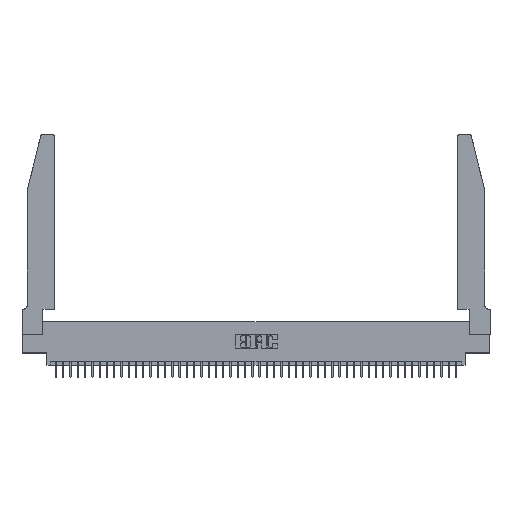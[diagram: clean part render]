
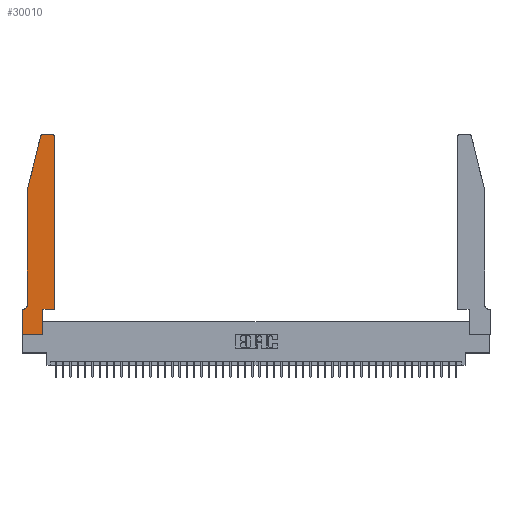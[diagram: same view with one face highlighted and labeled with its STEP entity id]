
A CAD part, top view. The second image highlights one B-rep face of the part: STEP entity #30010.
In plain terms, the highlighted planar face has unit normal (0, 0, 1).
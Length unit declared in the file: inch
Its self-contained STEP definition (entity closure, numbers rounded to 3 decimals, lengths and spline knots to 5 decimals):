
#52 = CARTESIAN_POINT ( 'NONE',  ( 0.4205, 2.75, 0.37 ) ) ;
#206 = VECTOR ( 'NONE', #19448, 39.37008 ) ;
#231 = VECTOR ( 'NONE', #16104, 39.37008 ) ;
#525 = LINE ( 'NONE', #16899, #36993 ) ;
#2098 = EDGE_CURVE ( 'NONE', #26644, #42607, #46910, .T. ) ;
#2677 = DIRECTION ( 'NONE',  ( 0., 0., -1. ) ) ;
#2873 = CARTESIAN_POINT ( 'NONE',  ( 0., 0., 0.37 ) ) ;
#5115 = VERTEX_POINT ( 'NONE', #46144 ) ;
#5498 = CARTESIAN_POINT ( 'NONE',  ( 0.284, 2.75, 0.37 ) ) ;
#6002 = AXIS2_PLACEMENT_3D ( 'NONE', #24562, #2677, #28212 ) ;
#6531 = ORIENTED_EDGE ( 'NONE', *, *, #21358, .T. ) ;
#7014 = CARTESIAN_POINT ( 'NONE',  ( 0., 0.35, 0.37 ) ) ;
#8141 = DIRECTION ( 'NONE',  ( 0., 1., 0. ) ) ;
#8501 = DIRECTION ( 'NONE',  ( 1., 0., 0. ) ) ;
#8911 = LINE ( 'NONE', #37451, #206 ) ;
#9303 = ORIENTED_EDGE ( 'NONE', *, *, #23251, .T. ) ;
#9736 = DIRECTION ( 'NONE',  ( 1., 0., 0. ) ) ;
#9850 = CARTESIAN_POINT ( 'NONE',  ( 0.0055, 0.35, 0.37 ) ) ;
#10050 = CARTESIAN_POINT ( 'NONE',  ( 0.4505, 2.72, 0.37 ) ) ;
#10442 = DIRECTION ( 'NONE',  ( -0.239, -0.971, 0. ) ) ;
#10679 = DIRECTION ( 'NONE',  ( 1., 0., 0. ) ) ;
#12460 = CARTESIAN_POINT ( 'NONE',  ( 0.2605, 2.75, 0.37 ) ) ;
#12537 = LINE ( 'NONE', #18976, #39134 ) ;
#13450 = CARTESIAN_POINT ( 'NONE',  ( 0.2865, 0., 0.37 ) ) ;
#15538 = VERTEX_POINT ( 'NONE', #2873 ) ;
#16104 = DIRECTION ( 'NONE',  ( -1., 0., 0. ) ) ;
#16208 = VERTEX_POINT ( 'NONE', #10050 ) ;
#16347 = CARTESIAN_POINT ( 'NONE',  ( 0.284, 2.72, 0.37 ) ) ;
#16579 = LINE ( 'NONE', #35060, #44237 ) ;
#16899 = CARTESIAN_POINT ( 'NONE',  ( 0., 0., 0.37 ) ) ;
#17254 = DIRECTION ( 'NONE',  ( 0., 0., 1. ) ) ;
#17348 = ORIENTED_EDGE ( 'NONE', *, *, #21017, .T. ) ;
#17384 = EDGE_CURVE ( 'NONE', #24950, #5115, #42437, .T. ) ;
#18054 = CARTESIAN_POINT ( 'NONE',  ( 0.2865, 0.35, 0.37 ) ) ;
#18840 = ORIENTED_EDGE ( 'NONE', *, *, #28044, .T. ) ;
#18976 = CARTESIAN_POINT ( 'NONE',  ( 0.2865, 0.35, 0.37 ) ) ;
#19448 = DIRECTION ( 'NONE',  ( -1., 0., 0. ) ) ;
#19461 = CIRCLE ( 'NONE', #28819, 0.03 ) ;
#19808 = ORIENTED_EDGE ( 'NONE', *, *, #28953, .T. ) ;
#20025 = DIRECTION ( 'NONE',  ( 1., 0., 0. ) ) ;
#20196 = VERTEX_POINT ( 'NONE', #38527 ) ;
#20366 = CARTESIAN_POINT ( 'NONE',  ( 0., 0.35, 0.37 ) ) ;
#20923 = LINE ( 'NONE', #12460, #231 ) ;
#21017 = EDGE_CURVE ( 'NONE', #16208, #32148, #25119, .T. ) ;
#21186 = EDGE_LOOP ( 'NONE', ( #9303, #39780, #45059, #41513, #21850, #19808, #25173, #21881, #6531, #23293, #18840, #17348 ) ) ;
#21194 = LINE ( 'NONE', #42920, #38115 ) ;
#21358 = EDGE_CURVE ( 'NONE', #45138, #24950, #12537, .T. ) ;
#21850 = ORIENTED_EDGE ( 'NONE', *, *, #23458, .T. ) ;
#21881 = ORIENTED_EDGE ( 'NONE', *, *, #25416, .T. ) ;
#23251 = EDGE_CURVE ( 'NONE', #32148, #41330, #20923, .T. ) ;
#23293 = ORIENTED_EDGE ( 'NONE', *, *, #17384, .T. ) ;
#23458 = EDGE_CURVE ( 'NONE', #20196, #37422, #41261, .T. ) ;
#24562 = CARTESIAN_POINT ( 'NONE',  ( 0.0055, 0.42, 0.37 ) ) ;
#24950 = VERTEX_POINT ( 'NONE', #18054 ) ;
#25119 = CIRCLE ( 'NONE', #32746, 0.03 ) ;
#25173 = ORIENTED_EDGE ( 'NONE', *, *, #37398, .T. ) ;
#25416 = EDGE_CURVE ( 'NONE', #15538, #45138, #525, .T. ) ;
#25746 = CARTESIAN_POINT ( 'NONE',  ( 0.4505, 0.35, 0.37 ) ) ;
#26644 = VERTEX_POINT ( 'NONE', #45790 ) ;
#27238 = VECTOR ( 'NONE', #29379, 39.37008 ) ;
#28044 = EDGE_CURVE ( 'NONE', #5115, #16208, #29495, .T. ) ;
#28212 = DIRECTION ( 'NONE',  ( -1., 0., 0. ) ) ;
#28576 = CARTESIAN_POINT ( 'NONE',  ( 0.0755, 2., 0.37 ) ) ;
#28819 = AXIS2_PLACEMENT_3D ( 'NONE', #16347, #41618, #20025 ) ;
#28953 = EDGE_CURVE ( 'NONE', #37422, #33259, #8911, .T. ) ;
#29379 = DIRECTION ( 'NONE',  ( 0., 1., 0. ) ) ;
#29495 = LINE ( 'NONE', #25746, #27238 ) ;
#30010 = ADVANCED_FACE ( 'NONE', ( #46660 ), #46669, .T. ) ;
#30124 = VECTOR ( 'NONE', #10442, 39.37008 ) ;
#30301 = CARTESIAN_POINT ( 'NONE',  ( 0.4505, 0.35, 0.37 ) ) ;
#31161 = AXIS2_PLACEMENT_3D ( 'NONE', #7014, #32446, #10679 ) ;
#32148 = VERTEX_POINT ( 'NONE', #52 ) ;
#32446 = DIRECTION ( 'NONE',  ( 0., 0., 1. ) ) ;
#32746 = AXIS2_PLACEMENT_3D ( 'NONE', #38884, #17254, #42492 ) ;
#33259 = VERTEX_POINT ( 'NONE', #20366 ) ;
#34064 = VECTOR ( 'NONE', #8501, 39.37008 ) ;
#35060 = CARTESIAN_POINT ( 'NONE',  ( 0., 0., 0.37 ) ) ;
#36844 = EDGE_CURVE ( 'NONE', #42607, #20196, #21194, .T. ) ;
#36993 = VECTOR ( 'NONE', #9736, 39.37008 ) ;
#37398 = EDGE_CURVE ( 'NONE', #33259, #15538, #16579, .T. ) ;
#37422 = VERTEX_POINT ( 'NONE', #9850 ) ;
#37451 = CARTESIAN_POINT ( 'NONE',  ( 0.0755, 0.35, 0.37 ) ) ;
#38115 = VECTOR ( 'NONE', #46518, 39.37008 ) ;
#38527 = CARTESIAN_POINT ( 'NONE',  ( 0.0755, 0.42, 0.37 ) ) ;
#38648 = DIRECTION ( 'NONE',  ( 0., -1., 0. ) ) ;
#38884 = CARTESIAN_POINT ( 'NONE',  ( 0.4205, 2.72, 0.37 ) ) ;
#39134 = VECTOR ( 'NONE', #8141, 39.37008 ) ;
#39780 = ORIENTED_EDGE ( 'NONE', *, *, #40326, .T. ) ;
#40326 = EDGE_CURVE ( 'NONE', #41330, #26644, #19461, .T. ) ;
#41261 = CIRCLE ( 'NONE', #6002, 0.07 ) ;
#41327 = CARTESIAN_POINT ( 'NONE',  ( 0.0755, 2., 0.37 ) ) ;
#41330 = VERTEX_POINT ( 'NONE', #5498 ) ;
#41513 = ORIENTED_EDGE ( 'NONE', *, *, #36844, .T. ) ;
#41618 = DIRECTION ( 'NONE',  ( 0., 0., 1. ) ) ;
#42437 = LINE ( 'NONE', #30301, #34064 ) ;
#42492 = DIRECTION ( 'NONE',  ( 1., 0., 0. ) ) ;
#42607 = VERTEX_POINT ( 'NONE', #41327 ) ;
#42920 = CARTESIAN_POINT ( 'NONE',  ( 0.0755, 2., 0.37 ) ) ;
#44237 = VECTOR ( 'NONE', #38648, 39.37008 ) ;
#45059 = ORIENTED_EDGE ( 'NONE', *, *, #2098, .T. ) ;
#45138 = VERTEX_POINT ( 'NONE', #13450 ) ;
#45790 = CARTESIAN_POINT ( 'NONE',  ( 0.25487, 2.72718, 0.37 ) ) ;
#46144 = CARTESIAN_POINT ( 'NONE',  ( 0.4505, 0.35, 0.37 ) ) ;
#46518 = DIRECTION ( 'NONE',  ( 0., -1., 0. ) ) ;
#46660 = FACE_OUTER_BOUND ( 'NONE', #21186, .T. ) ;
#46669 = PLANE ( 'NONE',  #31161 ) ;
#46910 = LINE ( 'NONE', #28576, #30124 ) ;
